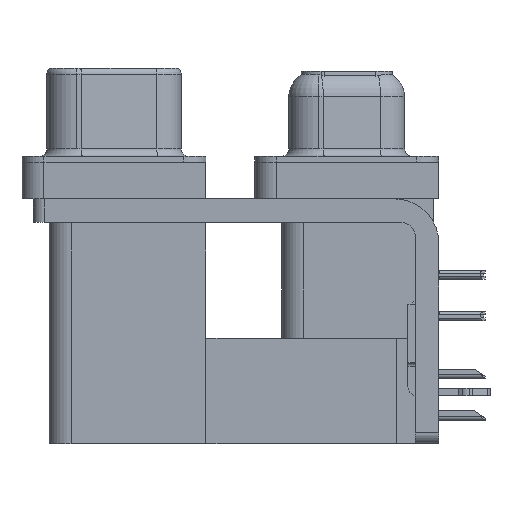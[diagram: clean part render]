
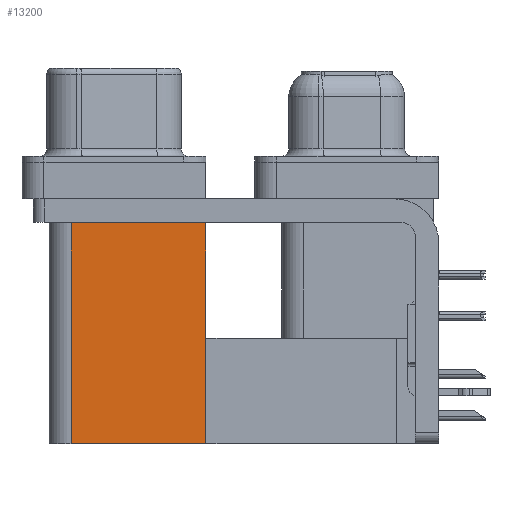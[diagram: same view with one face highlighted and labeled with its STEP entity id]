
A CAD part, left-side view. The second image highlights one B-rep face of the part: STEP entity #13200.
In plain terms, the highlighted planar face has unit normal (-1, 0, 0).
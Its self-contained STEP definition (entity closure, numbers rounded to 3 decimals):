
#36 = DIRECTION ( 'NONE',  ( 0., 0., 1. ) ) ;
#330 = EDGE_CURVE ( 'NONE', #6606, #22033, #43133, .T. ) ;
#1438 = EDGE_CURVE ( 'NONE', #12219, #22033, #36554, .T. ) ;
#1595 = VECTOR ( 'NONE', #19056, 1000. ) ;
#2782 = EDGE_CURVE ( 'NONE', #32482, #6606, #8493, .T. ) ;
#4389 = CARTESIAN_POINT ( 'NONE',  ( 3.765, 9.6, -2.5 ) ) ;
#6606 = VERTEX_POINT ( 'NONE', #4389 ) ;
#7083 = ORIENTED_EDGE ( 'NONE', *, *, #41358, .F. ) ;
#7652 = DIRECTION ( 'NONE',  ( 0., 0., -1. ) ) ;
#8493 = LINE ( 'NONE', #38609, #1595 ) ;
#9992 = DIRECTION ( 'NONE',  ( 0., 1., 0. ) ) ;
#11799 = FACE_OUTER_BOUND ( 'NONE', #22386, .T. ) ;
#11974 = VECTOR ( 'NONE', #26883, 1000. ) ;
#12219 = VERTEX_POINT ( 'NONE', #25258 ) ;
#13200 = ADVANCED_FACE ( 'NONE', ( #11799 ), #28539, .F. ) ;
#17206 = ORIENTED_EDGE ( 'NONE', *, *, #330, .T. ) ;
#17226 = ORIENTED_EDGE ( 'NONE', *, *, #2782, .T. ) ;
#17533 = DIRECTION ( 'NONE',  ( 1., 0., 0. ) ) ;
#19056 = DIRECTION ( 'NONE',  ( 0., 0., 1. ) ) ;
#20317 = CARTESIAN_POINT ( 'NONE',  ( 3.765, 9.6, -19.2 ) ) ;
#22033 = VERTEX_POINT ( 'NONE', #27514 ) ;
#22386 = EDGE_LOOP ( 'NONE', ( #17206, #31580, #7083, #17226 ) ) ;
#24626 = AXIS2_PLACEMENT_3D ( 'NONE', #34248, #17533, #7652 ) ;
#25258 = CARTESIAN_POINT ( 'NONE',  ( 3.765, 18.8, -19.2 ) ) ;
#26006 = CARTESIAN_POINT ( 'NONE',  ( 3.765, 9.6, -2.5 ) ) ;
#26883 = DIRECTION ( 'NONE',  ( 0., 1., 0. ) ) ;
#27514 = CARTESIAN_POINT ( 'NONE',  ( 3.765, 18.8, -2.5 ) ) ;
#28539 = PLANE ( 'NONE',  #24626 ) ;
#31580 = ORIENTED_EDGE ( 'NONE', *, *, #1438, .F. ) ;
#32482 = VERTEX_POINT ( 'NONE', #20317 ) ;
#34248 = CARTESIAN_POINT ( 'NONE',  ( 3.765, 9.6, -19.2 ) ) ;
#35773 = VECTOR ( 'NONE', #9992, 1000. ) ;
#36554 = LINE ( 'NONE', #43358, #42962 ) ;
#38609 = CARTESIAN_POINT ( 'NONE',  ( 3.765, 9.6, -19.2 ) ) ;
#40093 = LINE ( 'NONE', #43396, #35773 ) ;
#41358 = EDGE_CURVE ( 'NONE', #32482, #12219, #40093, .T. ) ;
#42962 = VECTOR ( 'NONE', #36, 1000. ) ;
#43133 = LINE ( 'NONE', #26006, #11974 ) ;
#43358 = CARTESIAN_POINT ( 'NONE',  ( 3.765, 18.8, -19.2 ) ) ;
#43396 = CARTESIAN_POINT ( 'NONE',  ( 3.765, 9.6, -19.2 ) ) ;
